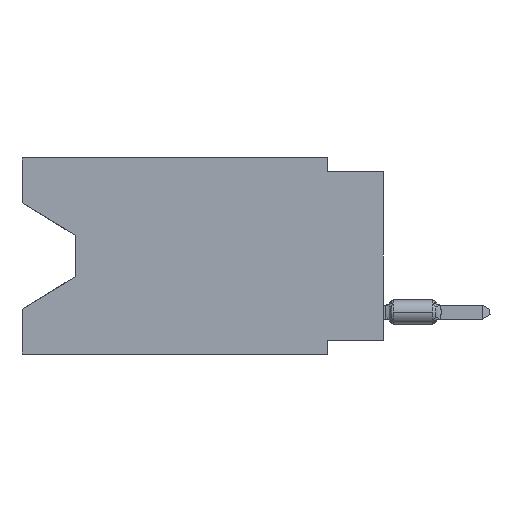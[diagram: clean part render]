
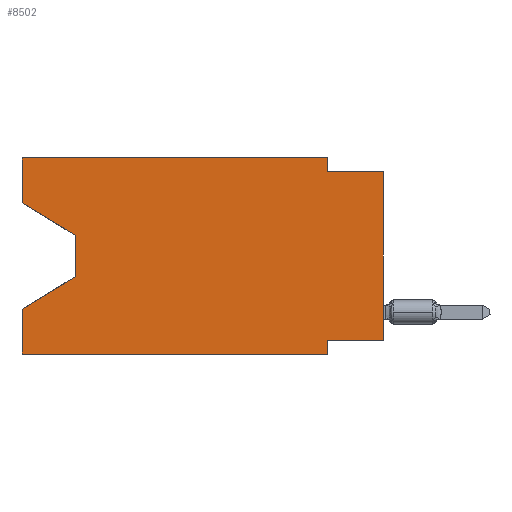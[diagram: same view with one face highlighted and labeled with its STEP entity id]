
A CAD part, left-side view. The second image highlights one B-rep face of the part: STEP entity #8502.
In plain terms, the highlighted planar face has unit normal (-1, 0, 0).
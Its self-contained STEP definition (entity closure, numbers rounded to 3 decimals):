
#141 = CARTESIAN_POINT ( 'NONE',  ( 0., 16.383, 0. ) ) ;
#1734 = CARTESIAN_POINT ( 'NONE',  ( 0., 16.383, 0. ) ) ;
#2075 = EDGE_CURVE ( 'NONE', #78812, #38928, #21931, .T. ) ;
#2694 = LINE ( 'NONE', #3856, #8076 ) ;
#3856 = CARTESIAN_POINT ( 'NONE',  ( 0., 0., -8.255 ) ) ;
#5106 = LINE ( 'NONE', #141, #35581 ) ;
#5168 = ORIENTED_EDGE ( 'NONE', *, *, #13336, .F. ) ;
#5887 = LINE ( 'NONE', #24331, #44156 ) ;
#6515 = LINE ( 'NONE', #105455, #107500 ) ;
#6592 = DIRECTION ( 'NONE',  ( 0., 0., 1. ) ) ;
#6622 = CARTESIAN_POINT ( 'NONE',  ( 0., 2.54, -8.255 ) ) ;
#8076 = VECTOR ( 'NONE', #111723, 1000. ) ;
#8502 = ADVANCED_FACE ( 'NONE', ( #45257 ), #55965, .F. ) ;
#13336 = EDGE_CURVE ( 'NONE', #92531, #57433, #99498, .T. ) ;
#15499 = ORIENTED_EDGE ( 'NONE', *, *, #97992, .T. ) ;
#18247 = CARTESIAN_POINT ( 'NONE',  ( 0., 16.383, -6.852 ) ) ;
#19029 = DIRECTION ( 'NONE',  ( 0., 0., -1. ) ) ;
#21418 = DIRECTION ( 'NONE',  ( 0., 0., -1. ) ) ;
#21931 = LINE ( 'NONE', #83947, #111726 ) ;
#22633 = LINE ( 'NONE', #63982, #66302 ) ;
#24331 = CARTESIAN_POINT ( 'NONE',  ( 0., 16.383, -8.89 ) ) ;
#27167 = CARTESIAN_POINT ( 'NONE',  ( 0., 2.54, -8.89 ) ) ;
#27902 = CARTESIAN_POINT ( 'NONE',  ( 0., 2.54, -0.635 ) ) ;
#29544 = EDGE_CURVE ( 'NONE', #61306, #69830, #5106, .T. ) ;
#33680 = VERTEX_POINT ( 'NONE', #84504 ) ;
#34833 = CARTESIAN_POINT ( 'NONE',  ( 0., 13.97, -3.505 ) ) ;
#35581 = VECTOR ( 'NONE', #62101, 1000. ) ;
#35657 = ORIENTED_EDGE ( 'NONE', *, *, #61721, .T. ) ;
#36916 = DIRECTION ( 'NONE',  ( 1., 0., 0. ) ) ;
#38765 = DIRECTION ( 'NONE',  ( 0., 0., -1. ) ) ;
#38928 = VERTEX_POINT ( 'NONE', #18247 ) ;
#39092 = CARTESIAN_POINT ( 'NONE',  ( 0., 16.383, 0. ) ) ;
#39674 = LINE ( 'NONE', #39092, #51995 ) ;
#40246 = AXIS2_PLACEMENT_3D ( 'NONE', #1734, #36916, #81620 ) ;
#40969 = EDGE_CURVE ( 'NONE', #69830, #92531, #22633, .T. ) ;
#41889 = CARTESIAN_POINT ( 'NONE',  ( 0., 2.54, 0. ) ) ;
#42771 = ORIENTED_EDGE ( 'NONE', *, *, #45416, .F. ) ;
#43413 = CARTESIAN_POINT ( 'NONE',  ( 0., 13.97, -5.385 ) ) ;
#44156 = VECTOR ( 'NONE', #113180, 1000. ) ;
#45257 = FACE_OUTER_BOUND ( 'NONE', #58295, .T. ) ;
#45416 = EDGE_CURVE ( 'NONE', #73479, #97716, #2694, .T. ) ;
#47975 = ORIENTED_EDGE ( 'NONE', *, *, #2075, .T. ) ;
#48742 = VERTEX_POINT ( 'NONE', #27167 ) ;
#49872 = ORIENTED_EDGE ( 'NONE', *, *, #73796, .T. ) ;
#50497 = EDGE_CURVE ( 'NONE', #57433, #107071, #84211, .T. ) ;
#51903 = VERTEX_POINT ( 'NONE', #34833 ) ;
#51995 = VECTOR ( 'NONE', #76052, 1000. ) ;
#52096 = VECTOR ( 'NONE', #19029, 1000. ) ;
#52382 = DIRECTION ( 'NONE',  ( 0., -0.855, -0.519 ) ) ;
#52816 = ORIENTED_EDGE ( 'NONE', *, *, #50497, .F. ) ;
#54711 = ORIENTED_EDGE ( 'NONE', *, *, #29544, .F. ) ;
#55965 = PLANE ( 'NONE',  #40246 ) ;
#56581 = ORIENTED_EDGE ( 'NONE', *, *, #107302, .F. ) ;
#57433 = VERTEX_POINT ( 'NONE', #27902 ) ;
#58295 = EDGE_LOOP ( 'NONE', ( #35657, #15499, #47975, #59781, #49872, #56581, #42771, #103336, #52816, #5168, #111382, #54711 ) ) ;
#59781 = ORIENTED_EDGE ( 'NONE', *, *, #117292, .F. ) ;
#61306 = VERTEX_POINT ( 'NONE', #77746 ) ;
#61721 = EDGE_CURVE ( 'NONE', #61306, #51903, #6515, .T. ) ;
#62101 = DIRECTION ( 'NONE',  ( 0., 0., 1. ) ) ;
#62406 = VECTOR ( 'NONE', #38765, 1000. ) ;
#63982 = CARTESIAN_POINT ( 'NONE',  ( 0., 16.383, 0. ) ) ;
#66302 = VECTOR ( 'NONE', #76302, 1000. ) ;
#66628 = DIRECTION ( 'NONE',  ( 0., 0.855, -0.519 ) ) ;
#69830 = VERTEX_POINT ( 'NONE', #98964 ) ;
#73479 = VERTEX_POINT ( 'NONE', #98353 ) ;
#73796 = EDGE_CURVE ( 'NONE', #33680, #48742, #5887, .T. ) ;
#74684 = CARTESIAN_POINT ( 'NONE',  ( 0., 0., -0.635 ) ) ;
#76016 = EDGE_CURVE ( 'NONE', #73479, #107071, #87634, .T. ) ;
#76052 = DIRECTION ( 'NONE',  ( 0., 0., 1. ) ) ;
#76302 = DIRECTION ( 'NONE',  ( 0., -1., 0. ) ) ;
#77746 = CARTESIAN_POINT ( 'NONE',  ( 0., 16.383, -2.038 ) ) ;
#78812 = VERTEX_POINT ( 'NONE', #43413 ) ;
#81620 = DIRECTION ( 'NONE',  ( 0., 0., -1. ) ) ;
#83947 = CARTESIAN_POINT ( 'NONE',  ( 0., 13.97, -5.385 ) ) ;
#84211 = LINE ( 'NONE', #74684, #106785 ) ;
#84504 = CARTESIAN_POINT ( 'NONE',  ( 0., 16.383, -8.89 ) ) ;
#86178 = VECTOR ( 'NONE', #6592, 1000. ) ;
#87634 = LINE ( 'NONE', #95415, #86178 ) ;
#92531 = VERTEX_POINT ( 'NONE', #41889 ) ;
#92564 = DIRECTION ( 'NONE',  ( 0., -1., 0. ) ) ;
#93345 = CARTESIAN_POINT ( 'NONE',  ( 0., 0., -0.635 ) ) ;
#95415 = CARTESIAN_POINT ( 'NONE',  ( 0., 0., 0. ) ) ;
#97716 = VERTEX_POINT ( 'NONE', #6622 ) ;
#97992 = EDGE_CURVE ( 'NONE', #51903, #78812, #103062, .T. ) ;
#98353 = CARTESIAN_POINT ( 'NONE',  ( 0., 0., -8.255 ) ) ;
#98964 = CARTESIAN_POINT ( 'NONE',  ( 0., 16.383, 0. ) ) ;
#99498 = LINE ( 'NONE', #107830, #52096 ) ;
#101945 = CARTESIAN_POINT ( 'NONE',  ( 0., 2.54, -8.89 ) ) ;
#103062 = LINE ( 'NONE', #109670, #113884 ) ;
#103336 = ORIENTED_EDGE ( 'NONE', *, *, #76016, .T. ) ;
#105455 = CARTESIAN_POINT ( 'NONE',  ( 0., 16.383, -2.038 ) ) ;
#106785 = VECTOR ( 'NONE', #92564, 1000. ) ;
#107071 = VERTEX_POINT ( 'NONE', #93345 ) ;
#107302 = EDGE_CURVE ( 'NONE', #97716, #48742, #113808, .T. ) ;
#107500 = VECTOR ( 'NONE', #52382, 1000. ) ;
#107830 = CARTESIAN_POINT ( 'NONE',  ( 0., 2.54, 0. ) ) ;
#109670 = CARTESIAN_POINT ( 'NONE',  ( 0., 13.97, -3.505 ) ) ;
#111382 = ORIENTED_EDGE ( 'NONE', *, *, #40969, .F. ) ;
#111723 = DIRECTION ( 'NONE',  ( 0., 1., 0. ) ) ;
#111726 = VECTOR ( 'NONE', #66628, 1000. ) ;
#113180 = DIRECTION ( 'NONE',  ( 0., -1., 0. ) ) ;
#113808 = LINE ( 'NONE', #101945, #62406 ) ;
#113884 = VECTOR ( 'NONE', #21418, 1000. ) ;
#117292 = EDGE_CURVE ( 'NONE', #33680, #38928, #39674, .T. ) ;
